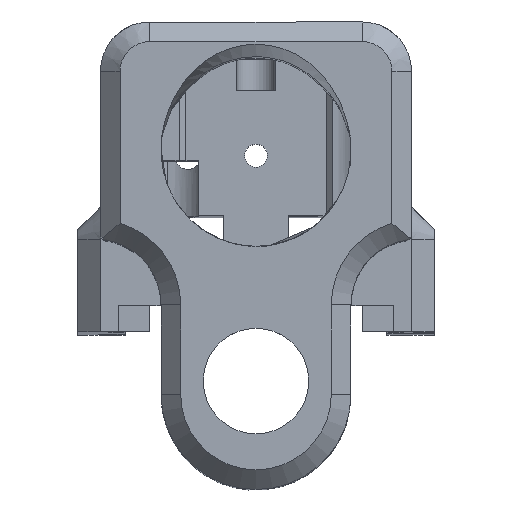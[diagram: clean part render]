
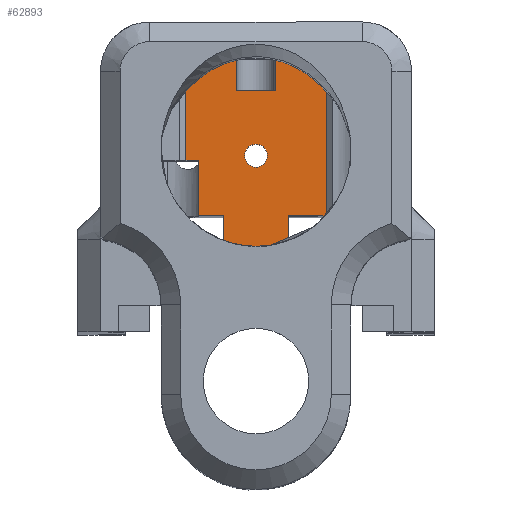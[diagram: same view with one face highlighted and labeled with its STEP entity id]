
A CAD part, top view. The second image highlights one B-rep face of the part: STEP entity #62893.
In plain terms, the highlighted planar face has unit normal (0, 0, 1).
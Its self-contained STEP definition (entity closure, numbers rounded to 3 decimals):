
#489 = ORIENTED_EDGE ( 'NONE', *, *, #33843, .T. ) ;
#1608 = VERTEX_POINT ( 'NONE', #54594 ) ;
#1957 = FACE_OUTER_BOUND ( 'NONE', #87837, .T. ) ;
#2038 = VECTOR ( 'NONE', #14750, 1000. ) ;
#2104 = DIRECTION ( 'NONE',  ( 0., 1., 0. ) ) ;
#2594 = CARTESIAN_POINT ( 'NONE',  ( -0.889, -10.16, -126.492 ) ) ;
#4051 = EDGE_CURVE ( 'NONE', #70189, #1608, #85086, .T. ) ;
#4843 = EDGE_CURVE ( 'NONE', #42684, #45238, #98263, .T. ) ;
#4892 = CARTESIAN_POINT ( 'NONE',  ( -1.524, -5.08, -126.492 ) ) ;
#6752 = EDGE_CURVE ( 'NONE', #45238, #67221, #21753, .T. ) ;
#7425 = VERTEX_POINT ( 'NONE', #79546 ) ;
#8123 = EDGE_CURVE ( 'NONE', #99859, #67221, #100275, .T. ) ;
#9231 = VERTEX_POINT ( 'NONE', #17141 ) ;
#10537 = DIRECTION ( 'NONE',  ( 0., 0., 1. ) ) ;
#11562 = DIRECTION ( 'NONE',  ( 0., 1., 0. ) ) ;
#12804 = CARTESIAN_POINT ( 'NONE',  ( 5.436, 0., -126.492 ) ) ;
#13156 = VECTOR ( 'NONE', #22633, 1000. ) ;
#13528 = LINE ( 'NONE', #42622, #101620 ) ;
#14750 = DIRECTION ( 'NONE',  ( 0., -1., 0. ) ) ;
#15156 = CARTESIAN_POINT ( 'NONE',  ( -2.489, -14.834, -126.492 ) ) ;
#17141 = CARTESIAN_POINT ( 'NONE',  ( 1.524, -5.08, -126.492 ) ) ;
#17959 = ORIENTED_EDGE ( 'NONE', *, *, #4843, .F. ) ;
#19108 = VECTOR ( 'NONE', #47148, 1000. ) ;
#19315 = VERTEX_POINT ( 'NONE', #87766 ) ;
#19626 = DIRECTION ( 'NONE',  ( 0., 0., 1. ) ) ;
#20324 = EDGE_CURVE ( 'NONE', #100283, #99263, #70068, .T. ) ;
#20519 = EDGE_CURVE ( 'NONE', #79321, #19315, #54055, .T. ) ;
#21753 = LINE ( 'NONE', #12804, #19108 ) ;
#22633 = DIRECTION ( 'NONE',  ( 1., 0., 0. ) ) ;
#23074 = CARTESIAN_POINT ( 'NONE',  ( -5.436, -14.834, -126.492 ) ) ;
#23544 = CARTESIAN_POINT ( 'NONE',  ( 2.489, -14.834, -126.492 ) ) ;
#24921 = ORIENTED_EDGE ( 'NONE', *, *, #31691, .T. ) ;
#25848 = ORIENTED_EDGE ( 'NONE', *, *, #98174, .T. ) ;
#27373 = DIRECTION ( 'NONE',  ( 1., 0., 0. ) ) ;
#27584 = ORIENTED_EDGE ( 'NONE', *, *, #20519, .F. ) ;
#29389 = VERTEX_POINT ( 'NONE', #78604 ) ;
#29890 = VECTOR ( 'NONE', #76259, 1000. ) ;
#31691 = EDGE_CURVE ( 'NONE', #7425, #19315, #35371, .T. ) ;
#31864 = CARTESIAN_POINT ( 'NONE',  ( -2.489, -18.72, -126.492 ) ) ;
#32531 = ORIENTED_EDGE ( 'NONE', *, *, #4051, .F. ) ;
#33843 = EDGE_CURVE ( 'NONE', #107098, #86096, #35819, .T. ) ;
#33993 = AXIS2_PLACEMENT_3D ( 'NONE', #61642, #10537, #70196 ) ;
#34690 = ORIENTED_EDGE ( 'NONE', *, *, #6752, .F. ) ;
#35371 = LINE ( 'NONE', #104254, #78125 ) ;
#35819 = LINE ( 'NONE', #108030, #13156 ) ;
#36019 = VERTEX_POINT ( 'NONE', #15156 ) ;
#38770 = ORIENTED_EDGE ( 'NONE', *, *, #56754, .F. ) ;
#40245 = CARTESIAN_POINT ( 'NONE',  ( -4.445, -10.516, -126.492 ) ) ;
#40278 = ORIENTED_EDGE ( 'NONE', *, *, #60386, .F. ) ;
#41114 = DIRECTION ( 'NONE',  ( 1., 0., 0. ) ) ;
#42593 = AXIS2_PLACEMENT_3D ( 'NONE', #70739, #19626, #79303 ) ;
#42622 = CARTESIAN_POINT ( 'NONE',  ( -5.436, 0., -126.492 ) ) ;
#42684 = VERTEX_POINT ( 'NONE', #52260 ) ;
#43090 = ORIENTED_EDGE ( 'NONE', *, *, #73894, .T. ) ;
#45069 = LINE ( 'NONE', #23074, #110360 ) ;
#45238 = VERTEX_POINT ( 'NONE', #94412 ) ;
#45559 = CARTESIAN_POINT ( 'NONE',  ( -5.436, 0., -126.492 ) ) ;
#47148 = DIRECTION ( 'NONE',  ( 0., -1., 0. ) ) ;
#47831 = DIRECTION ( 'NONE',  ( 1., 0., 0. ) ) ;
#49652 = EDGE_CURVE ( 'NONE', #100283, #29389, #82547, .T. ) ;
#49703 = CARTESIAN_POINT ( 'NONE',  ( -5.436, 0., -126.492 ) ) ;
#50706 = VECTOR ( 'NONE', #60783, 1000. ) ;
#52236 = CARTESIAN_POINT ( 'NONE',  ( 2.489, 0., -126.492 ) ) ;
#52260 = CARTESIAN_POINT ( 'NONE',  ( 1.524, 0., -126.492 ) ) ;
#52405 = CARTESIAN_POINT ( 'NONE',  ( 5.436, -14.834, -126.492 ) ) ;
#52936 = VECTOR ( 'NONE', #41114, 1000. ) ;
#53964 = DIRECTION ( 'NONE',  ( -1., 0., 0. ) ) ;
#54055 = LINE ( 'NONE', #69910, #99384 ) ;
#54594 = CARTESIAN_POINT ( 'NONE',  ( 0.889, -10.16, -126.492 ) ) ;
#56754 = EDGE_CURVE ( 'NONE', #1608, #70189, #78227, .T. ) ;
#57668 = CARTESIAN_POINT ( 'NONE',  ( -5.436, -14.834, -126.492 ) ) ;
#57942 = CARTESIAN_POINT ( 'NONE',  ( -5.436, 0., -126.492 ) ) ;
#60386 = EDGE_CURVE ( 'NONE', #7425, #9231, #74453, .T. ) ;
#60470 = CARTESIAN_POINT ( 'NONE',  ( -2.489, 0., -126.492 ) ) ;
#60783 = DIRECTION ( 'NONE',  ( 0., 1., 0. ) ) ;
#61041 = CARTESIAN_POINT ( 'NONE',  ( 2.489, -18.72, -126.492 ) ) ;
#61642 = CARTESIAN_POINT ( 'NONE',  ( 0., -10.16, -126.492 ) ) ;
#62692 = DIRECTION ( 'NONE',  ( 0., 0., -1. ) ) ;
#62893 = ADVANCED_FACE ( 'NONE', ( #1957, #67292 ), #96614, .F. ) ;
#66275 = DIRECTION ( 'NONE',  ( 1., 0., 0. ) ) ;
#67221 = VERTEX_POINT ( 'NONE', #52405 ) ;
#67292 = FACE_BOUND ( 'NONE', #94010, .T. ) ;
#67763 = ORIENTED_EDGE ( 'NONE', *, *, #49652, .F. ) ;
#68704 = AXIS2_PLACEMENT_3D ( 'NONE', #45559, #62692, #11562 ) ;
#69910 = CARTESIAN_POINT ( 'NONE',  ( -5.436, 0., -126.492 ) ) ;
#70068 = LINE ( 'NONE', #91270, #2038 ) ;
#70189 = VERTEX_POINT ( 'NONE', #2594 ) ;
#70196 = DIRECTION ( 'NONE',  ( 0., 1., 0. ) ) ;
#70739 = CARTESIAN_POINT ( 'NONE',  ( 0., -10.16, -126.492 ) ) ;
#71815 = VECTOR ( 'NONE', #47831, 1000. ) ;
#73348 = LINE ( 'NONE', #52236, #50706 ) ;
#73894 = EDGE_CURVE ( 'NONE', #86096, #99859, #73348, .T. ) ;
#74453 = LINE ( 'NONE', #4892, #71815 ) ;
#76259 = DIRECTION ( 'NONE',  ( 0., 1., 0. ) ) ;
#78125 = VECTOR ( 'NONE', #2104, 1000. ) ;
#78227 = CIRCLE ( 'NONE', #33993, 0.889 ) ;
#78604 = CARTESIAN_POINT ( 'NONE',  ( -5.436, -10.516, -126.492 ) ) ;
#79303 = DIRECTION ( 'NONE',  ( 0., 1., 0. ) ) ;
#79321 = VERTEX_POINT ( 'NONE', #57942 ) ;
#79546 = CARTESIAN_POINT ( 'NONE',  ( -1.524, -5.08, -126.492 ) ) ;
#79667 = ORIENTED_EDGE ( 'NONE', *, *, #20324, .T. ) ;
#79922 = VECTOR ( 'NONE', #53964, 1000. ) ;
#82159 = ORIENTED_EDGE ( 'NONE', *, *, #89031, .T. ) ;
#82547 = LINE ( 'NONE', #87493, #79922 ) ;
#85086 = CIRCLE ( 'NONE', #42593, 0.889 ) ;
#86096 = VERTEX_POINT ( 'NONE', #61041 ) ;
#87493 = CARTESIAN_POINT ( 'NONE',  ( -5.436, -10.516, -126.492 ) ) ;
#87766 = CARTESIAN_POINT ( 'NONE',  ( -1.524, 0., -126.492 ) ) ;
#87837 = EDGE_LOOP ( 'NONE', ( #17959, #109675, #40278, #24921, #27584, #82159, #67763, #79667, #25848, #99245, #489, #43090, #95593, #34690 ) ) ;
#89031 = EDGE_CURVE ( 'NONE', #79321, #29389, #13528, .T. ) ;
#91270 = CARTESIAN_POINT ( 'NONE',  ( -4.445, 0., -126.492 ) ) ;
#91395 = DIRECTION ( 'NONE',  ( 1., 0., 0. ) ) ;
#93710 = DIRECTION ( 'NONE',  ( 0., -1., 0. ) ) ;
#94010 = EDGE_LOOP ( 'NONE', ( #32531, #38770 ) ) ;
#94412 = CARTESIAN_POINT ( 'NONE',  ( 5.436, 0., -126.492 ) ) ;
#94732 = EDGE_CURVE ( 'NONE', #9231, #42684, #100699, .T. ) ;
#95593 = ORIENTED_EDGE ( 'NONE', *, *, #8123, .T. ) ;
#96614 = PLANE ( 'NONE',  #68704 ) ;
#96823 = EDGE_CURVE ( 'NONE', #36019, #107098, #103983, .T. ) ;
#97608 = VECTOR ( 'NONE', #66275, 1000. ) ;
#98174 = EDGE_CURVE ( 'NONE', #99263, #36019, #45069, .T. ) ;
#98263 = LINE ( 'NONE', #49703, #52936 ) ;
#98638 = VECTOR ( 'NONE', #103311, 1000. ) ;
#99245 = ORIENTED_EDGE ( 'NONE', *, *, #96823, .T. ) ;
#99263 = VERTEX_POINT ( 'NONE', #100778 ) ;
#99384 = VECTOR ( 'NONE', #27373, 1000. ) ;
#99859 = VERTEX_POINT ( 'NONE', #23544 ) ;
#100275 = LINE ( 'NONE', #57668, #97608 ) ;
#100283 = VERTEX_POINT ( 'NONE', #40245 ) ;
#100699 = LINE ( 'NONE', #110153, #29890 ) ;
#100778 = CARTESIAN_POINT ( 'NONE',  ( -4.445, -14.834, -126.492 ) ) ;
#101620 = VECTOR ( 'NONE', #93710, 1000. ) ;
#103311 = DIRECTION ( 'NONE',  ( 0., -1., 0. ) ) ;
#103983 = LINE ( 'NONE', #60470, #98638 ) ;
#104254 = CARTESIAN_POINT ( 'NONE',  ( -1.524, -5.08, -126.492 ) ) ;
#107098 = VERTEX_POINT ( 'NONE', #31864 ) ;
#108030 = CARTESIAN_POINT ( 'NONE',  ( -13.844, -18.72, -126.492 ) ) ;
#109675 = ORIENTED_EDGE ( 'NONE', *, *, #94732, .F. ) ;
#110153 = CARTESIAN_POINT ( 'NONE',  ( 1.524, -5.08, -126.492 ) ) ;
#110360 = VECTOR ( 'NONE', #91395, 1000. ) ;
